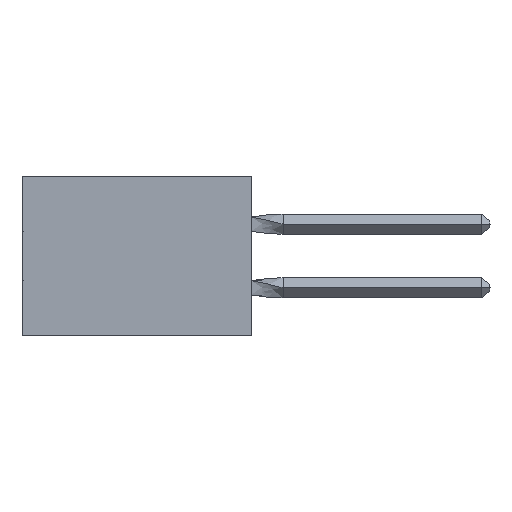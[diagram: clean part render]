
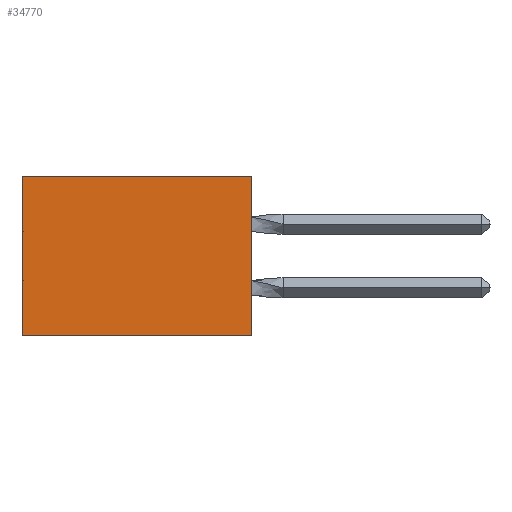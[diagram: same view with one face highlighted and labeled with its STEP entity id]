
A CAD part, left-side view. The second image highlights one B-rep face of the part: STEP entity #34770.
In plain terms, the highlighted planar face has unit normal (-1, 0, 0).
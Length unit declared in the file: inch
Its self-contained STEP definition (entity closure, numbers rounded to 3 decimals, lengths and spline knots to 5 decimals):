
#178 = CARTESIAN_POINT ( 'NONE',  ( 0.305, 0., 0. ) ) ;
#237 = LINE ( 'NONE', #178, #50953 ) ;
#370 = VECTOR ( 'NONE', #51067, 39.37008 ) ;
#1173 = CARTESIAN_POINT ( 'NONE',  ( 0.305, 0., 0. ) ) ;
#1859 = CARTESIAN_POINT ( 'NONE',  ( 0.305, 0., -0.5 ) ) ;
#2378 = ORIENTED_EDGE ( 'NONE', *, *, #31939, .F. ) ;
#3560 = LINE ( 'NONE', #27100, #21320 ) ;
#5787 = ORIENTED_EDGE ( 'NONE', *, *, #22755, .T. ) ;
#8626 = LINE ( 'NONE', #42933, #370 ) ;
#11622 = CARTESIAN_POINT ( 'NONE',  ( 0.305, 0., -0.5 ) ) ;
#12324 = ORIENTED_EDGE ( 'NONE', *, *, #51205, .F. ) ;
#12599 = DIRECTION ( 'NONE',  ( 0., 1., 0. ) ) ;
#14667 = ORIENTED_EDGE ( 'NONE', *, *, #42023, .T. ) ;
#14910 = CARTESIAN_POINT ( 'NONE',  ( 0.305, 0.72, 0. ) ) ;
#16036 = DIRECTION ( 'NONE',  ( 1., 0., 0. ) ) ;
#18782 = VECTOR ( 'NONE', #22909, 39.37008 ) ;
#20623 = VERTEX_POINT ( 'NONE', #14910 ) ;
#21320 = VECTOR ( 'NONE', #23764, 39.37008 ) ;
#21920 = EDGE_LOOP ( 'NONE', ( #14667, #2378, #12324, #5787 ) ) ;
#22755 = EDGE_CURVE ( 'NONE', #38514, #20623, #237, .T. ) ;
#22909 = DIRECTION ( 'NONE',  ( 0., 0., -1. ) ) ;
#23764 = DIRECTION ( 'NONE',  ( 0., 1., 0. ) ) ;
#27080 = CARTESIAN_POINT ( 'NONE',  ( 0.305, 0.72, -0.5 ) ) ;
#27100 = CARTESIAN_POINT ( 'NONE',  ( 0.305, 0., -0.5 ) ) ;
#30538 = AXIS2_PLACEMENT_3D ( 'NONE', #11622, #16036, #44038 ) ;
#31902 = PLANE ( 'NONE',  #30538 ) ;
#31939 = EDGE_CURVE ( 'NONE', #49238, #38098, #3560, .T. ) ;
#32371 = FACE_OUTER_BOUND ( 'NONE', #21920, .T. ) ;
#34770 = ADVANCED_FACE ( 'NONE', ( #32371 ), #31902, .F. ) ;
#38098 = VERTEX_POINT ( 'NONE', #27080 ) ;
#38514 = VERTEX_POINT ( 'NONE', #1173 ) ;
#42023 = EDGE_CURVE ( 'NONE', #20623, #38098, #8626, .T. ) ;
#42933 = CARTESIAN_POINT ( 'NONE',  ( 0.305, 0.72, -0.5 ) ) ;
#44038 = DIRECTION ( 'NONE',  ( 0., 0., -1. ) ) ;
#46992 = CARTESIAN_POINT ( 'NONE',  ( 0.305, 0., -0.5 ) ) ;
#47222 = LINE ( 'NONE', #46992, #18782 ) ;
#49238 = VERTEX_POINT ( 'NONE', #1859 ) ;
#50953 = VECTOR ( 'NONE', #12599, 39.37008 ) ;
#51067 = DIRECTION ( 'NONE',  ( 0., 0., -1. ) ) ;
#51205 = EDGE_CURVE ( 'NONE', #38514, #49238, #47222, .T. ) ;
